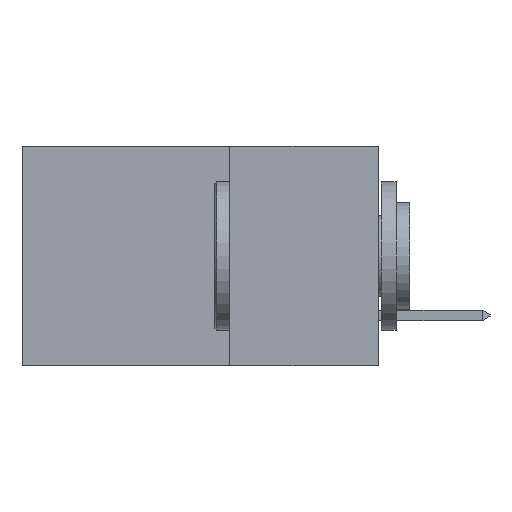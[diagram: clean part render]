
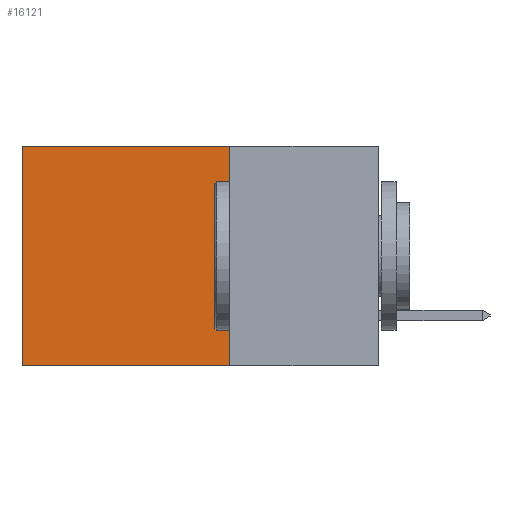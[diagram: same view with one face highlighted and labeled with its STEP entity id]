
A CAD part, left-side view. The second image highlights one B-rep face of the part: STEP entity #16121.
In plain terms, the highlighted planar face has unit normal (-1, 0, 0).
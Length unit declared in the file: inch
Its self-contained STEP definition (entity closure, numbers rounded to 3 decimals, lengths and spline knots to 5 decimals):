
#556 = CARTESIAN_POINT ( 'NONE',  ( 0.298, 0.25, 0. ) ) ;
#2116 = VERTEX_POINT ( 'NONE', #13027 ) ;
#2326 = DIRECTION ( 'NONE',  ( 0., 1., 0. ) ) ;
#3966 = VECTOR ( 'NONE', #12411, 39.37008 ) ;
#3989 = VECTOR ( 'NONE', #15494, 39.37008 ) ;
#4716 = PLANE ( 'NONE',  #16241 ) ;
#4854 = LINE ( 'NONE', #17790, #9603 ) ;
#6048 = CARTESIAN_POINT ( 'NONE',  ( 0.298, 0.25, 0. ) ) ;
#6784 = DIRECTION ( 'NONE',  ( 0., 0., -1. ) ) ;
#7180 = ORIENTED_EDGE ( 'NONE', *, *, #18649, .F. ) ;
#7367 = EDGE_CURVE ( 'NONE', #10569, #11240, #22860, .T. ) ;
#7674 = VERTEX_POINT ( 'NONE', #20758 ) ;
#9403 = LINE ( 'NONE', #13554, #3989 ) ;
#9603 = VECTOR ( 'NONE', #12078, 39.37008 ) ;
#10468 = CARTESIAN_POINT ( 'NONE',  ( 0.298, 0.25, 0. ) ) ;
#10569 = VERTEX_POINT ( 'NONE', #6048 ) ;
#11240 = VERTEX_POINT ( 'NONE', #23280 ) ;
#11340 = FACE_OUTER_BOUND ( 'NONE', #12740, .T. ) ;
#12078 = DIRECTION ( 'NONE',  ( 0., 1., 0. ) ) ;
#12411 = DIRECTION ( 'NONE',  ( 0., 0., -1. ) ) ;
#12740 = EDGE_LOOP ( 'NONE', ( #13318, #15370, #7180, #13880 ) ) ;
#12779 = VECTOR ( 'NONE', #2326, 39.37008 ) ;
#12970 = EDGE_CURVE ( 'NONE', #11240, #7674, #9403, .T. ) ;
#13027 = CARTESIAN_POINT ( 'NONE',  ( 0.298, 0.25, -0.37 ) ) ;
#13318 = ORIENTED_EDGE ( 'NONE', *, *, #12970, .T. ) ;
#13554 = CARTESIAN_POINT ( 'NONE',  ( 0.298, 0.6, 0. ) ) ;
#13880 = ORIENTED_EDGE ( 'NONE', *, *, #7367, .T. ) ;
#15370 = ORIENTED_EDGE ( 'NONE', *, *, #20010, .F. ) ;
#15494 = DIRECTION ( 'NONE',  ( 0., 0., -1. ) ) ;
#16121 = ADVANCED_FACE ( 'NONE', ( #11340 ), #4716, .F. ) ;
#16241 = AXIS2_PLACEMENT_3D ( 'NONE', #556, #18411, #6784 ) ;
#17790 = CARTESIAN_POINT ( 'NONE',  ( 0.298, 0.25, -0.37 ) ) ;
#18083 = CARTESIAN_POINT ( 'NONE',  ( 0.298, 0.25, 0. ) ) ;
#18411 = DIRECTION ( 'NONE',  ( 1., 0., 0. ) ) ;
#18649 = EDGE_CURVE ( 'NONE', #10569, #2116, #19559, .T. ) ;
#19559 = LINE ( 'NONE', #10468, #3966 ) ;
#20010 = EDGE_CURVE ( 'NONE', #2116, #7674, #4854, .T. ) ;
#20758 = CARTESIAN_POINT ( 'NONE',  ( 0.298, 0.6, -0.37 ) ) ;
#22860 = LINE ( 'NONE', #18083, #12779 ) ;
#23280 = CARTESIAN_POINT ( 'NONE',  ( 0.298, 0.6, 0. ) ) ;
